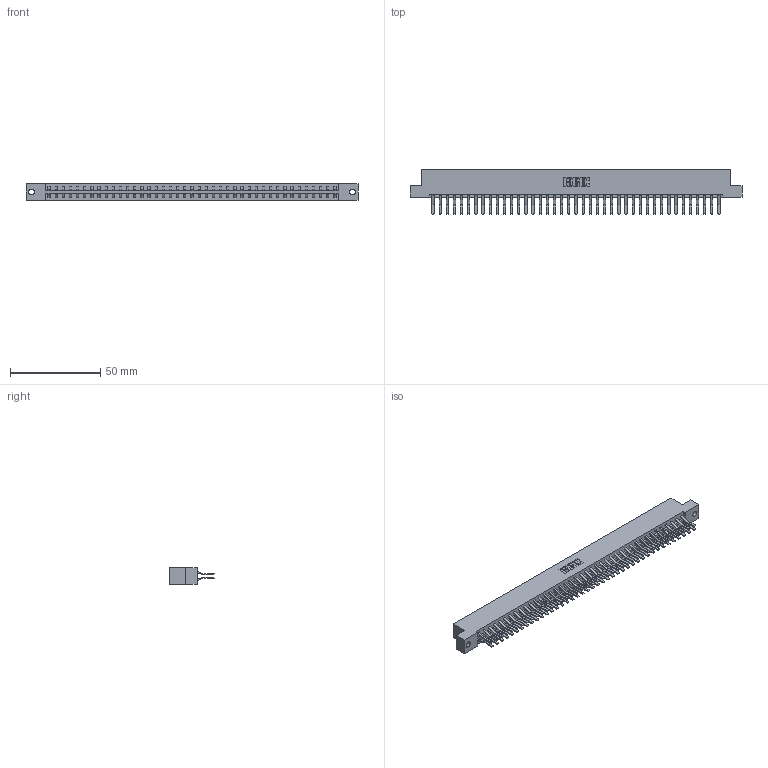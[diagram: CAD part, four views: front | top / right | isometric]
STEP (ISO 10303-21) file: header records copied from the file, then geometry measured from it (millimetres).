
FILE_DESCRIPTION (( 'STEP AP203' ), '1' );
FILE_NAME ('833-082-560-202.STEP', '2020-06-06T00:34:13', ( '' ), ( '' ), 'SwSTEP 2.0', 'SolidWorks 2020', '' );
FILE_SCHEMA (( 'CONFIG_CONTROL_DESIGN' ));
Length unit declared in the file: inch
Products named in the file (3): 833 Part_Flush - .128 Dia; 345-292-001_560 Tail; 833-082-560-202
Assembly tree (83 placements, depth 2):
  833-082-560-202
    833 Part_Flush - .128 Dia
    345-292-001_560 Tail  x82
Bounding box: 184 x 24.78 x 9.4 mm (x, y, z)
Volume: 19276.6 mm3; surface area: 24038.8 mm2
Topology: 83 solids, 83 shells, 4542 faces, 13513 edges, 8898 vertices
Faces by surface type: plane 3022, cylinder 1520
Entity records: 26597 total; most frequent: CARTESIAN_POINT 4410, ORIENTED_EDGE 4346, DIRECTION 3773, EDGE_CURVE 2173, LINE 2041, VECTOR 2041, VERTEX_POINT 1446, AXIS2_PLACEMENT_3D 866
